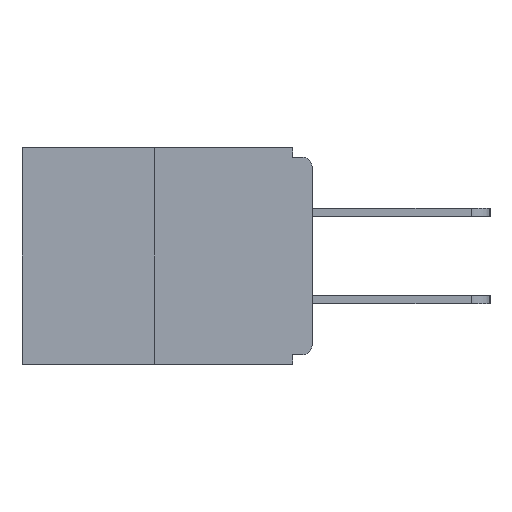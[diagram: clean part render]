
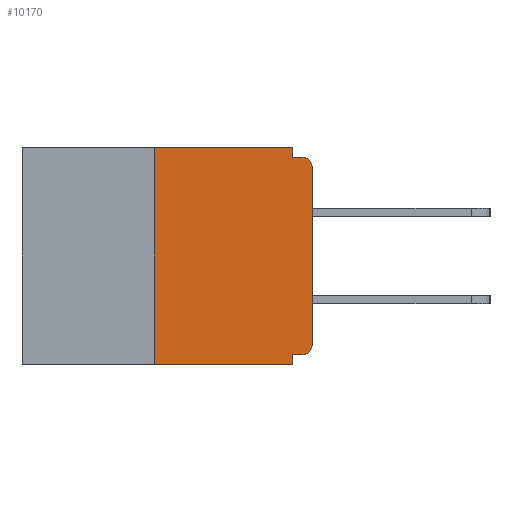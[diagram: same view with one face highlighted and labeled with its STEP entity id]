
A CAD part, left-side view. The second image highlights one B-rep face of the part: STEP entity #10170.
In plain terms, the highlighted planar face has unit normal (-1, 0, 0).
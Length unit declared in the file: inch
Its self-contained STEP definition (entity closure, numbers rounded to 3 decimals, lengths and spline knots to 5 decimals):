
#41 = ORIENTED_EDGE ( 'NONE', *, *, #13000, .F. ) ;
#590 = DIRECTION ( 'NONE',  ( 0., 0., 1. ) ) ;
#950 = CARTESIAN_POINT ( 'NONE',  ( 0., 0.46, 0. ) ) ;
#994 = PLANE ( 'NONE',  #7661 ) ;
#1048 = ORIENTED_EDGE ( 'NONE', *, *, #7080, .F. ) ;
#1185 = DIRECTION ( 'NONE',  ( 0., 0., -1. ) ) ;
#1194 = ORIENTED_EDGE ( 'NONE', *, *, #8921, .T. ) ;
#1265 = DIRECTION ( 'NONE',  ( 0., 0., -1. ) ) ;
#1288 = CARTESIAN_POINT ( 'NONE',  ( 0., 0.25, -0.343 ) ) ;
#1398 = EDGE_CURVE ( 'NONE', #1656, #8599, #15157, .T. ) ;
#1403 = LINE ( 'NONE', #7859, #10513 ) ;
#1656 = VERTEX_POINT ( 'NONE', #5439 ) ;
#1677 = DIRECTION ( 'NONE',  ( 0., 0., 1. ) ) ;
#2099 = DIRECTION ( 'NONE',  ( 0., -1., 0. ) ) ;
#2170 = VERTEX_POINT ( 'NONE', #8343 ) ;
#2403 = LINE ( 'NONE', #6710, #11933 ) ;
#2530 = CARTESIAN_POINT ( 'NONE',  ( 0., 0.031, -0.328 ) ) ;
#2657 = VECTOR ( 'NONE', #9392, 39.37008 ) ;
#2764 = CARTESIAN_POINT ( 'NONE',  ( 0., 0.25, 0. ) ) ;
#2806 = LINE ( 'NONE', #2764, #9412 ) ;
#3220 = EDGE_CURVE ( 'NONE', #2170, #12561, #13600, .T. ) ;
#3254 = EDGE_CURVE ( 'NONE', #9790, #12463, #9344, .T. ) ;
#3270 = DIRECTION ( 'NONE',  ( 0., 0., -1. ) ) ;
#3828 = VERTEX_POINT ( 'NONE', #3960 ) ;
#3960 = CARTESIAN_POINT ( 'NONE',  ( 0., 0.031, -0.015 ) ) ;
#4334 = CARTESIAN_POINT ( 'NONE',  ( 0., 0.031, -0.343 ) ) ;
#4567 = CARTESIAN_POINT ( 'NONE',  ( 0., 0., -0.328 ) ) ;
#4584 = AXIS2_PLACEMENT_3D ( 'NONE', #10289, #8116, #3270 ) ;
#4621 = CARTESIAN_POINT ( 'NONE',  ( 0., 0., -0.03 ) ) ;
#4728 = CARTESIAN_POINT ( 'NONE',  ( 0., 0.031, -0.343 ) ) ;
#4743 = VECTOR ( 'NONE', #11497, 39.37008 ) ;
#5069 = ORIENTED_EDGE ( 'NONE', *, *, #11967, .F. ) ;
#5155 = EDGE_CURVE ( 'NONE', #12561, #13304, #12034, .T. ) ;
#5439 = CARTESIAN_POINT ( 'NONE',  ( 0., 0.25, 0. ) ) ;
#5513 = CARTESIAN_POINT ( 'NONE',  ( 0., 0.015, -0.015 ) ) ;
#5852 = CARTESIAN_POINT ( 'NONE',  ( 0., 0.015, -0.328 ) ) ;
#6057 = EDGE_LOOP ( 'NONE', ( #13300, #41, #1194, #11562, #5069, #10659, #6588, #11028, #1048, #13867 ) ) ;
#6588 = ORIENTED_EDGE ( 'NONE', *, *, #3220, .T. ) ;
#6710 = CARTESIAN_POINT ( 'NONE',  ( 0., 0.46, -0.343 ) ) ;
#6800 = DIRECTION ( 'NONE',  ( 0., -1., 0. ) ) ;
#6959 = CARTESIAN_POINT ( 'NONE',  ( 0., 0.031, 0. ) ) ;
#6983 = CARTESIAN_POINT ( 'NONE',  ( 0., 0.031, 0. ) ) ;
#7080 = EDGE_CURVE ( 'NONE', #3828, #13304, #1403, .T. ) ;
#7554 = VERTEX_POINT ( 'NONE', #5852 ) ;
#7661 = AXIS2_PLACEMENT_3D ( 'NONE', #950, #9147, #13722 ) ;
#7859 = CARTESIAN_POINT ( 'NONE',  ( 0., 0., -0.015 ) ) ;
#8116 = DIRECTION ( 'NONE',  ( -1., 0., 0. ) ) ;
#8343 = CARTESIAN_POINT ( 'NONE',  ( 0., 0., -0.313 ) ) ;
#8599 = VERTEX_POINT ( 'NONE', #6983 ) ;
#8919 = VECTOR ( 'NONE', #6800, 39.37008 ) ;
#8921 = EDGE_CURVE ( 'NONE', #11700, #12463, #2403, .T. ) ;
#9147 = DIRECTION ( 'NONE',  ( 1., 0., 0. ) ) ;
#9344 = LINE ( 'NONE', #4728, #11377 ) ;
#9392 = DIRECTION ( 'NONE',  ( 0., 1., 0. ) ) ;
#9412 = VECTOR ( 'NONE', #1677, 39.37008 ) ;
#9510 = CARTESIAN_POINT ( 'NONE',  ( 0., 0.015, -0.03 ) ) ;
#9658 = EDGE_CURVE ( 'NONE', #8599, #3828, #14116, .T. ) ;
#9790 = VERTEX_POINT ( 'NONE', #2530 ) ;
#9886 = CARTESIAN_POINT ( 'NONE',  ( 0., 0., 0. ) ) ;
#10170 = ADVANCED_FACE ( 'NONE', ( #10974 ), #994, .F. ) ;
#10186 = LINE ( 'NONE', #4567, #2657 ) ;
#10289 = CARTESIAN_POINT ( 'NONE',  ( 0., 0.015, -0.313 ) ) ;
#10513 = VECTOR ( 'NONE', #2099, 39.37008 ) ;
#10659 = ORIENTED_EDGE ( 'NONE', *, *, #13959, .T. ) ;
#10974 = FACE_OUTER_BOUND ( 'NONE', #6057, .T. ) ;
#11028 = ORIENTED_EDGE ( 'NONE', *, *, #5155, .T. ) ;
#11377 = VECTOR ( 'NONE', #1185, 39.37008 ) ;
#11497 = DIRECTION ( 'NONE',  ( 0., 0., -1. ) ) ;
#11562 = ORIENTED_EDGE ( 'NONE', *, *, #3254, .F. ) ;
#11700 = VERTEX_POINT ( 'NONE', #1288 ) ;
#11933 = VECTOR ( 'NONE', #15061, 39.37008 ) ;
#11967 = EDGE_CURVE ( 'NONE', #7554, #9790, #10186, .T. ) ;
#12034 = CIRCLE ( 'NONE', #12353, 0.015 ) ;
#12353 = AXIS2_PLACEMENT_3D ( 'NONE', #9510, #14081, #1265 ) ;
#12463 = VERTEX_POINT ( 'NONE', #4334 ) ;
#12561 = VERTEX_POINT ( 'NONE', #4621 ) ;
#13000 = EDGE_CURVE ( 'NONE', #11700, #1656, #2806, .T. ) ;
#13300 = ORIENTED_EDGE ( 'NONE', *, *, #1398, .F. ) ;
#13304 = VERTEX_POINT ( 'NONE', #5513 ) ;
#13600 = LINE ( 'NONE', #9886, #14659 ) ;
#13722 = DIRECTION ( 'NONE',  ( 0., 0., -1. ) ) ;
#13778 = CARTESIAN_POINT ( 'NONE',  ( 0., 0.46, 0. ) ) ;
#13867 = ORIENTED_EDGE ( 'NONE', *, *, #9658, .F. ) ;
#13959 = EDGE_CURVE ( 'NONE', #7554, #2170, #14721, .T. ) ;
#14081 = DIRECTION ( 'NONE',  ( -1., 0., 0. ) ) ;
#14116 = LINE ( 'NONE', #6959, #4743 ) ;
#14659 = VECTOR ( 'NONE', #590, 39.37008 ) ;
#14721 = CIRCLE ( 'NONE', #4584, 0.015 ) ;
#15061 = DIRECTION ( 'NONE',  ( 0., -1., 0. ) ) ;
#15157 = LINE ( 'NONE', #13778, #8919 ) ;
